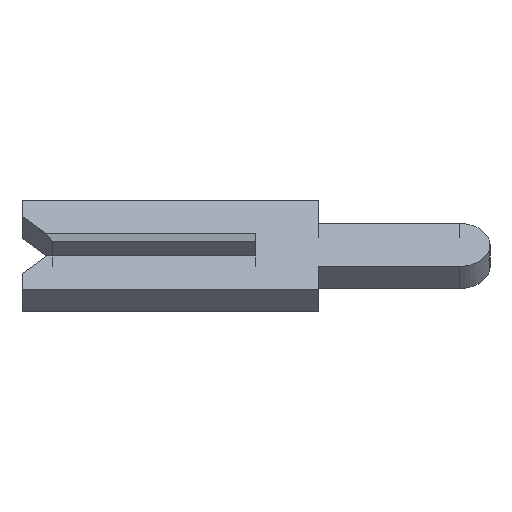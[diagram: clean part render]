
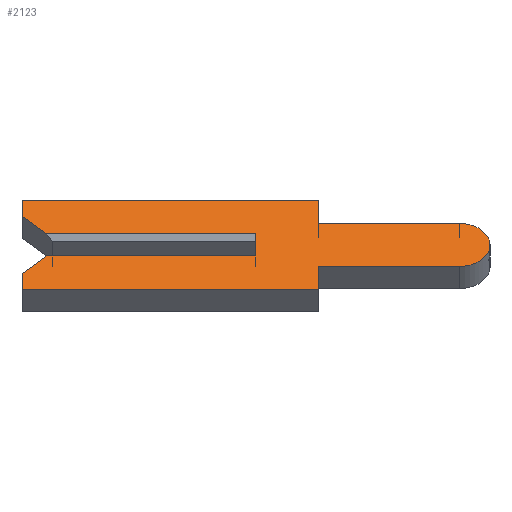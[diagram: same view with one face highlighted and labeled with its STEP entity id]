
A CAD part, left-side view. The second image highlights one B-rep face of the part: STEP entity #2123.
In plain terms, the highlighted face is planar.
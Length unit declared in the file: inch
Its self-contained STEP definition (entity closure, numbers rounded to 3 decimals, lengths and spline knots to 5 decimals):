
#5 = AXIS2_PLACEMENT_3D ( 'NONE', #913, #753, #201 ) ;
#18 = ORIENTED_EDGE ( 'NONE', *, *, #664, .F. ) ;
#48 = AXIS2_PLACEMENT_3D ( 'NONE', #935, #246, #756 ) ;
#64 = VERTEX_POINT ( 'NONE', #1297 ) ;
#95 = LINE ( 'NONE', #1293, #1831 ) ;
#143 = CARTESIAN_POINT ( 'NONE',  ( -0.01, 0.15, 0.04 ) ) ;
#149 = VECTOR ( 'NONE', #1966, 39.37008 ) ;
#201 = DIRECTION ( 'NONE',  ( 0., 0., -1. ) ) ;
#210 = CARTESIAN_POINT ( 'NONE',  ( -0.01, -0.1305, 0.0195 ) ) ;
#232 = ORIENTED_EDGE ( 'NONE', *, *, #2113, .F. ) ;
#235 = VECTOR ( 'NONE', #1533, 39.37008 ) ;
#245 = EDGE_CURVE ( 'NONE', #1317, #2046, #2141, .T. ) ;
#246 = DIRECTION ( 'NONE',  ( 1., 0., 0. ) ) ;
#259 = CARTESIAN_POINT ( 'NONE',  ( -0.01, 0.1305, -0.0065 ) ) ;
#268 = LINE ( 'NONE', #832, #1407 ) ;
#302 = VERTEX_POINT ( 'NONE', #561 ) ;
#305 = ORIENTED_EDGE ( 'NONE', *, *, #601, .F. ) ;
#359 = VERTEX_POINT ( 'NONE', #368 ) ;
#368 = CARTESIAN_POINT ( 'NONE',  ( -0.01, 0., 0.01 ) ) ;
#381 = VECTOR ( 'NONE', #1880, 39.37008 ) ;
#385 = PLANE ( 'NONE',  #5 ) ;
#415 = EDGE_CURVE ( 'NONE', #2162, #359, #1719, .T. ) ;
#468 = VECTOR ( 'NONE', #2324, 39.37008 ) ;
#492 = CARTESIAN_POINT ( 'NONE',  ( -0.01, 0.134, -0.01 ) ) ;
#504 = DIRECTION ( 'NONE',  ( 0., 0., -1. ) ) ;
#526 = LINE ( 'NONE', #1038, #468 ) ;
#536 = VERTEX_POINT ( 'NONE', #210 ) ;
#561 = CARTESIAN_POINT ( 'NONE',  ( -0.01, -0.1305, -0.0195 ) ) ;
#581 = CARTESIAN_POINT ( 'NONE',  ( -0.01, 0., 0.0065 ) ) ;
#601 = EDGE_CURVE ( 'NONE', #302, #1945, #914, .T. ) ;
#648 = DIRECTION ( 'NONE',  ( 0., 0., 1. ) ) ;
#664 = EDGE_CURVE ( 'NONE', #536, #302, #1389, .T. ) ;
#700 = VECTOR ( 'NONE', #808, 39.37008 ) ;
#714 = CARTESIAN_POINT ( 'NONE',  ( -0.01, 0.15, 0.026 ) ) ;
#718 = ORIENTED_EDGE ( 'NONE', *, *, #1399, .T. ) ;
#721 = CARTESIAN_POINT ( 'NONE',  ( -0.01, 0.15, -0.026 ) ) ;
#750 = DIRECTION ( 'NONE',  ( 0., 1., 0. ) ) ;
#753 = DIRECTION ( 'NONE',  ( 1., 0., 0. ) ) ;
#756 = DIRECTION ( 'NONE',  ( 0., 0., -1. ) ) ;
#808 = DIRECTION ( 'NONE',  ( 0., -0.707, 0.707 ) ) ;
#832 = CARTESIAN_POINT ( 'NONE',  ( -0.01, -0.04, -0.04 ) ) ;
#833 = EDGE_LOOP ( 'NONE', ( #718, #1229, #232, #1272, #2241, #1215, #1182, #305, #18, #2073, #1772, #930, #1718, #1736 ) ) ;
#856 = LINE ( 'NONE', #2309, #1360 ) ;
#879 = EDGE_CURVE ( 'NONE', #1983, #1515, #2306, .T. ) ;
#907 = CARTESIAN_POINT ( 'NONE',  ( -0.01, -0.04, 0.0195 ) ) ;
#913 = CARTESIAN_POINT ( 'NONE',  ( -0.01, -0.1305, 0. ) ) ;
#914 = LINE ( 'NONE', #1686, #1985 ) ;
#930 = ORIENTED_EDGE ( 'NONE', *, *, #1421, .F. ) ;
#935 = CARTESIAN_POINT ( 'NONE',  ( -0.01, -0.1305, 0. ) ) ;
#1038 = CARTESIAN_POINT ( 'NONE',  ( -0.01, 0.15, 0.04 ) ) ;
#1044 = CARTESIAN_POINT ( 'NONE',  ( -0.01, -0.04, -0.04 ) ) ;
#1055 = EDGE_CURVE ( 'NONE', #2046, #1983, #2154, .T. ) ;
#1071 = CARTESIAN_POINT ( 'NONE',  ( -0.01, 0.15, -0.04 ) ) ;
#1083 = CARTESIAN_POINT ( 'NONE',  ( -0.01, -0.04, 0.04 ) ) ;
#1107 = DIRECTION ( 'NONE',  ( 0., 0., -1. ) ) ;
#1125 = VERTEX_POINT ( 'NONE', #1175 ) ;
#1175 = CARTESIAN_POINT ( 'NONE',  ( -0.01, 0.134, 0.01 ) ) ;
#1182 = ORIENTED_EDGE ( 'NONE', *, *, #1356, .F. ) ;
#1215 = ORIENTED_EDGE ( 'NONE', *, *, #245, .F. ) ;
#1229 = ORIENTED_EDGE ( 'NONE', *, *, #415, .F. ) ;
#1231 = EDGE_CURVE ( 'NONE', #2163, #536, #2183, .T. ) ;
#1245 = VECTOR ( 'NONE', #1107, 39.37008 ) ;
#1272 = ORIENTED_EDGE ( 'NONE', *, *, #879, .F. ) ;
#1293 = CARTESIAN_POINT ( 'NONE',  ( -0.01, -0.1305, -0.01 ) ) ;
#1297 = CARTESIAN_POINT ( 'NONE',  ( -0.01, 0.15, 0.026 ) ) ;
#1317 = VERTEX_POINT ( 'NONE', #1044 ) ;
#1343 = VERTEX_POINT ( 'NONE', #143 ) ;
#1356 = EDGE_CURVE ( 'NONE', #1945, #1317, #268, .T. ) ;
#1360 = VECTOR ( 'NONE', #2149, 39.37008 ) ;
#1363 = VECTOR ( 'NONE', #750, 39.37008 ) ;
#1389 = CIRCLE ( 'NONE', #48, 0.0195 ) ;
#1399 = EDGE_CURVE ( 'NONE', #1125, #359, #856, .T. ) ;
#1407 = VECTOR ( 'NONE', #504, 39.37008 ) ;
#1421 = EDGE_CURVE ( 'NONE', #1343, #1806, #526, .T. ) ;
#1434 = FACE_OUTER_BOUND ( 'NONE', #833, .T. ) ;
#1467 = CARTESIAN_POINT ( 'NONE',  ( -0.01, -0.04, 0.04 ) ) ;
#1471 = CARTESIAN_POINT ( 'NONE',  ( -0.01, 0.15, -0.04 ) ) ;
#1503 = DIRECTION ( 'NONE',  ( 0., 1., 0. ) ) ;
#1515 = VERTEX_POINT ( 'NONE', #492 ) ;
#1533 = DIRECTION ( 'NONE',  ( 0., -1., 0. ) ) ;
#1556 = CARTESIAN_POINT ( 'NONE',  ( -0.01, 0.1305, 0.0065 ) ) ;
#1568 = EDGE_CURVE ( 'NONE', #1125, #64, #1572, .T. ) ;
#1572 = LINE ( 'NONE', #1556, #149 ) ;
#1601 = VECTOR ( 'NONE', #1816, 39.37008 ) ;
#1644 = EDGE_CURVE ( 'NONE', #64, #1343, #2152, .T. ) ;
#1664 = CARTESIAN_POINT ( 'NONE',  ( -0.01, 0., -0.01 ) ) ;
#1686 = CARTESIAN_POINT ( 'NONE',  ( -0.01, -0.04, -0.0195 ) ) ;
#1718 = ORIENTED_EDGE ( 'NONE', *, *, #1644, .F. ) ;
#1719 = LINE ( 'NONE', #581, #381 ) ;
#1736 = ORIENTED_EDGE ( 'NONE', *, *, #1568, .F. ) ;
#1772 = ORIENTED_EDGE ( 'NONE', *, *, #2171, .F. ) ;
#1776 = LINE ( 'NONE', #1467, #1245 ) ;
#1806 = VERTEX_POINT ( 'NONE', #1083 ) ;
#1809 = VECTOR ( 'NONE', #648, 39.37008 ) ;
#1816 = DIRECTION ( 'NONE',  ( 0., 0., 1. ) ) ;
#1831 = VECTOR ( 'NONE', #1837, 39.37008 ) ;
#1837 = DIRECTION ( 'NONE',  ( 0., -1., 0. ) ) ;
#1880 = DIRECTION ( 'NONE',  ( 0., 0., 1. ) ) ;
#1945 = VERTEX_POINT ( 'NONE', #1998 ) ;
#1966 = DIRECTION ( 'NONE',  ( 0., 0.707, 0.707 ) ) ;
#1983 = VERTEX_POINT ( 'NONE', #721 ) ;
#1985 = VECTOR ( 'NONE', #1503, 39.37008 ) ;
#1998 = CARTESIAN_POINT ( 'NONE',  ( -0.01, -0.04, -0.0195 ) ) ;
#2046 = VERTEX_POINT ( 'NONE', #1071 ) ;
#2073 = ORIENTED_EDGE ( 'NONE', *, *, #1231, .F. ) ;
#2113 = EDGE_CURVE ( 'NONE', #1515, #2162, #95, .T. ) ;
#2123 = ADVANCED_FACE ( 'NONE', ( #1434 ), #385, .F. ) ;
#2141 = LINE ( 'NONE', #1471, #1363 ) ;
#2149 = DIRECTION ( 'NONE',  ( 0., -1., 0. ) ) ;
#2152 = LINE ( 'NONE', #714, #1601 ) ;
#2154 = LINE ( 'NONE', #2293, #1809 ) ;
#2162 = VERTEX_POINT ( 'NONE', #1664 ) ;
#2163 = VERTEX_POINT ( 'NONE', #907 ) ;
#2171 = EDGE_CURVE ( 'NONE', #1806, #2163, #1776, .T. ) ;
#2183 = LINE ( 'NONE', #2303, #235 ) ;
#2241 = ORIENTED_EDGE ( 'NONE', *, *, #1055, .F. ) ;
#2293 = CARTESIAN_POINT ( 'NONE',  ( -0.01, 0.15, -0.026 ) ) ;
#2303 = CARTESIAN_POINT ( 'NONE',  ( -0.01, -0.04, 0.0195 ) ) ;
#2306 = LINE ( 'NONE', #259, #700 ) ;
#2309 = CARTESIAN_POINT ( 'NONE',  ( -0.01, 0.15, 0.01 ) ) ;
#2324 = DIRECTION ( 'NONE',  ( 0., -1., 0. ) ) ;
